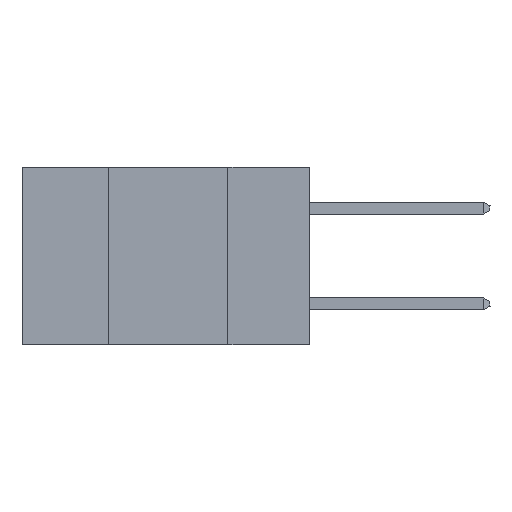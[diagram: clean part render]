
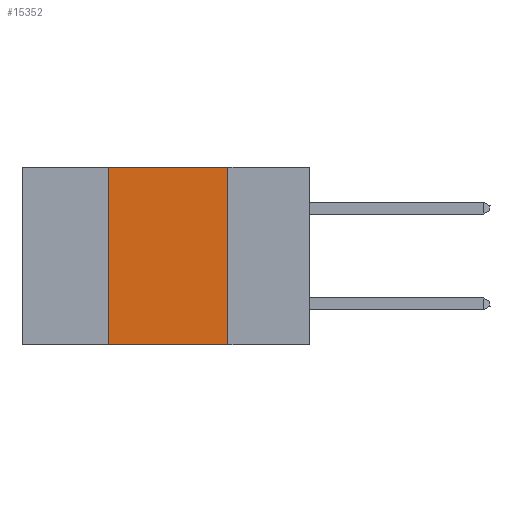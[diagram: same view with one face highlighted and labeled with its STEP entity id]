
A CAD part, left-side view. The second image highlights one B-rep face of the part: STEP entity #15352.
In plain terms, the highlighted planar face has unit normal (-1, 0, 0).
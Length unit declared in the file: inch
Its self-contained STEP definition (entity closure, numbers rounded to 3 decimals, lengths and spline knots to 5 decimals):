
#255 = CARTESIAN_POINT ( 'NONE',  ( 0., 0.17, -0.37 ) ) ;
#502 = CARTESIAN_POINT ( 'NONE',  ( 0., 0.6, 0. ) ) ;
#740 = DIRECTION ( 'NONE',  ( 1., 0., 0. ) ) ;
#944 = FACE_OUTER_BOUND ( 'NONE', #16554, .T. ) ;
#1022 = DIRECTION ( 'NONE',  ( 0., -1., 0. ) ) ;
#1763 = EDGE_CURVE ( 'NONE', #12257, #15431, #6326, .T. ) ;
#2488 = VECTOR ( 'NONE', #17935, 39.37008 ) ;
#2584 = AXIS2_PLACEMENT_3D ( 'NONE', #502, #740, #15034 ) ;
#2626 = LINE ( 'NONE', #15857, #7174 ) ;
#2743 = CARTESIAN_POINT ( 'NONE',  ( 0., 0.17, 0. ) ) ;
#2840 = CARTESIAN_POINT ( 'NONE',  ( 0., 0.17, 0. ) ) ;
#3672 = CARTESIAN_POINT ( 'NONE',  ( 0., 0.42, 0. ) ) ;
#4149 = DIRECTION ( 'NONE',  ( 0., 0., -1. ) ) ;
#4389 = ORIENTED_EDGE ( 'NONE', *, *, #1763, .F. ) ;
#4488 = EDGE_CURVE ( 'NONE', #12257, #11179, #2626, .T. ) ;
#4982 = ORIENTED_EDGE ( 'NONE', *, *, #14459, .F. ) ;
#5245 = CARTESIAN_POINT ( 'NONE',  ( 0., 0.42, 0. ) ) ;
#5529 = CARTESIAN_POINT ( 'NONE',  ( 0., 0.42, -0.37 ) ) ;
#6326 = LINE ( 'NONE', #3672, #2488 ) ;
#7123 = DIRECTION ( 'NONE',  ( 0., -1., 0. ) ) ;
#7174 = VECTOR ( 'NONE', #7123, 39.37008 ) ;
#8693 = ORIENTED_EDGE ( 'NONE', *, *, #12372, .F. ) ;
#8925 = VERTEX_POINT ( 'NONE', #2840 ) ;
#9426 = PLANE ( 'NONE',  #2584 ) ;
#9712 = CARTESIAN_POINT ( 'NONE',  ( 0., 0.6, 0. ) ) ;
#10478 = LINE ( 'NONE', #9712, #14325 ) ;
#11011 = VECTOR ( 'NONE', #4149, 39.37008 ) ;
#11179 = VERTEX_POINT ( 'NONE', #255 ) ;
#11713 = LINE ( 'NONE', #2743, #11011 ) ;
#12257 = VERTEX_POINT ( 'NONE', #5529 ) ;
#12372 = EDGE_CURVE ( 'NONE', #8925, #11179, #11713, .T. ) ;
#14325 = VECTOR ( 'NONE', #1022, 39.37008 ) ;
#14459 = EDGE_CURVE ( 'NONE', #15431, #8925, #10478, .T. ) ;
#15034 = DIRECTION ( 'NONE',  ( 0., 0., -1. ) ) ;
#15352 = ADVANCED_FACE ( 'NONE', ( #944 ), #9426, .F. ) ;
#15431 = VERTEX_POINT ( 'NONE', #5245 ) ;
#15466 = ORIENTED_EDGE ( 'NONE', *, *, #4488, .T. ) ;
#15857 = CARTESIAN_POINT ( 'NONE',  ( 0., 0.6, -0.37 ) ) ;
#16554 = EDGE_LOOP ( 'NONE', ( #8693, #4982, #4389, #15466 ) ) ;
#17935 = DIRECTION ( 'NONE',  ( 0., 0., 1. ) ) ;
